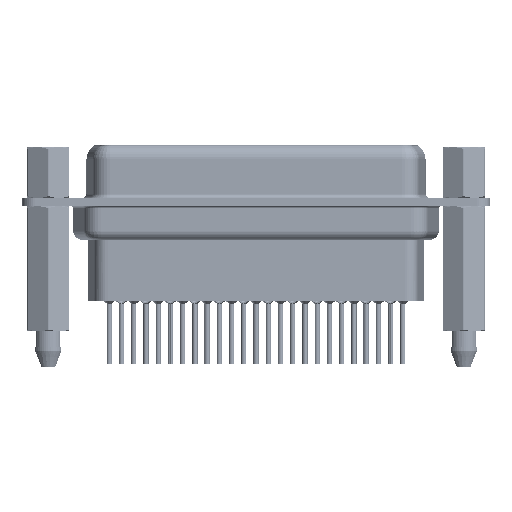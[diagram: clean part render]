
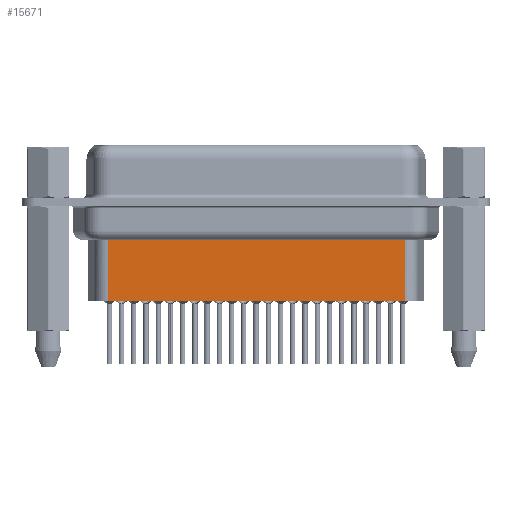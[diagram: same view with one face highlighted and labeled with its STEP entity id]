
A CAD part, front view. The second image highlights one B-rep face of the part: STEP entity #15671.
In plain terms, the highlighted planar face has unit normal (0, -1, 0).
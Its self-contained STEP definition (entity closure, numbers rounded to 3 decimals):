
#349 = LINE ( 'NONE', #11098, #21479 ) ;
#529 = EDGE_LOOP ( 'NONE', ( #5330, #13642, #6800, #25832 ) ) ;
#3832 = CARTESIAN_POINT ( 'NONE',  ( 6.706, -3.5, -3.1 ) ) ;
#5330 = ORIENTED_EDGE ( 'NONE', *, *, #24261, .F. ) ;
#6294 = VERTEX_POINT ( 'NONE', #16979 ) ;
#6672 = VERTEX_POINT ( 'NONE', #7168 ) ;
#6800 = ORIENTED_EDGE ( 'NONE', *, *, #23590, .T. ) ;
#7168 = CARTESIAN_POINT ( 'NONE',  ( 6.706, -3.5, -4.097 ) ) ;
#7250 = DIRECTION ( 'NONE',  ( 0., 0., -1. ) ) ;
#7302 = VERTEX_POINT ( 'NONE', #7460 ) ;
#7460 = CARTESIAN_POINT ( 'NONE',  ( 6.706, -3.5, -11.15 ) ) ;
#7540 = DIRECTION ( 'NONE',  ( 0., 0., -1. ) ) ;
#7609 = VECTOR ( 'NONE', #19556, 1000. ) ;
#8222 = AXIS2_PLACEMENT_3D ( 'NONE', #3832, #24592, #14264 ) ;
#8853 = CARTESIAN_POINT ( 'NONE',  ( 40.344, -3.5, -11.15 ) ) ;
#11098 = CARTESIAN_POINT ( 'NONE',  ( 6.459, -3.5, -4.097 ) ) ;
#11668 = CARTESIAN_POINT ( 'NONE',  ( 6.706, -3.5, -11.15 ) ) ;
#13642 = ORIENTED_EDGE ( 'NONE', *, *, #23711, .T. ) ;
#14088 = PLANE ( 'NONE',  #8222 ) ;
#14264 = DIRECTION ( 'NONE',  ( 1., 0., 0. ) ) ;
#15671 = ADVANCED_FACE ( 'NONE', ( #19587 ), #14088, .T. ) ;
#16979 = CARTESIAN_POINT ( 'NONE',  ( 40.344, -3.5, -4.097 ) ) ;
#17325 = LINE ( 'NONE', #11668, #7609 ) ;
#19473 = EDGE_CURVE ( 'NONE', #27898, #7302, #17325, .T. ) ;
#19556 = DIRECTION ( 'NONE',  ( -1., 0., 0. ) ) ;
#19587 = FACE_OUTER_BOUND ( 'NONE', #529, .T. ) ;
#21479 = VECTOR ( 'NONE', #29159, 1000. ) ;
#23590 = EDGE_CURVE ( 'NONE', #6672, #7302, #31411, .T. ) ;
#23711 = EDGE_CURVE ( 'NONE', #6294, #6672, #349, .T. ) ;
#24261 = EDGE_CURVE ( 'NONE', #6294, #27898, #27685, .T. ) ;
#24592 = DIRECTION ( 'NONE',  ( 0., -1., 0. ) ) ;
#25832 = ORIENTED_EDGE ( 'NONE', *, *, #19473, .F. ) ;
#26426 = VECTOR ( 'NONE', #7540, 1000. ) ;
#27578 = VECTOR ( 'NONE', #7250, 1000. ) ;
#27685 = LINE ( 'NONE', #30772, #27578 ) ;
#27898 = VERTEX_POINT ( 'NONE', #8853 ) ;
#29159 = DIRECTION ( 'NONE',  ( -1., 0., 0. ) ) ;
#30772 = CARTESIAN_POINT ( 'NONE',  ( 40.344, -3.5, -3.1 ) ) ;
#31411 = LINE ( 'NONE', #33803, #26426 ) ;
#33803 = CARTESIAN_POINT ( 'NONE',  ( 6.706, -3.5, -3.1 ) ) ;
